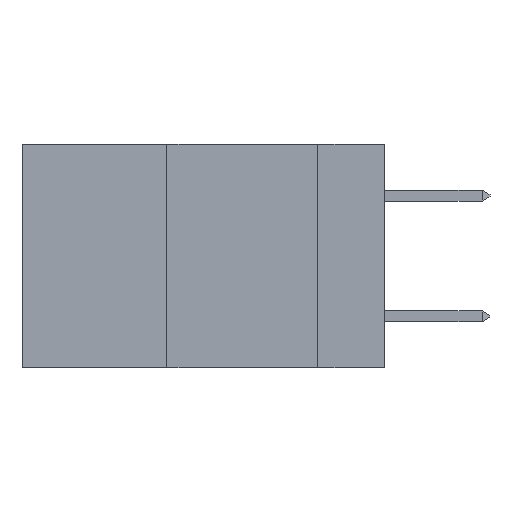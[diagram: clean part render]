
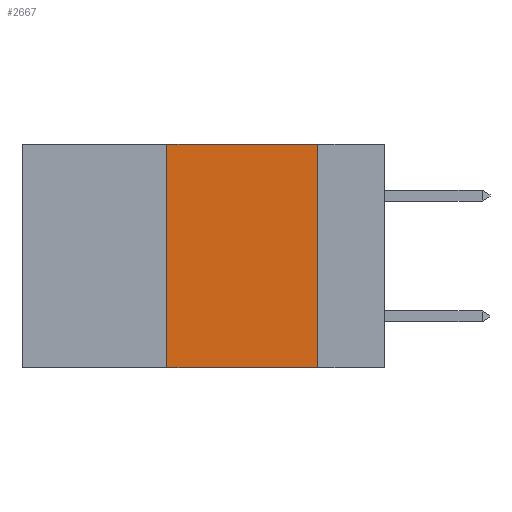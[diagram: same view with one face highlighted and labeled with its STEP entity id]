
A CAD part, left-side view. The second image highlights one B-rep face of the part: STEP entity #2667.
In plain terms, the highlighted planar face has unit normal (-1, 0, 0).
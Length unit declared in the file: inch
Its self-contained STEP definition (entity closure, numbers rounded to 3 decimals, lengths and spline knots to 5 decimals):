
#435 = LINE ( 'NONE', #2800, #4077 ) ;
#770 = AXIS2_PLACEMENT_3D ( 'NONE', #1539, #5183, #4234 ) ;
#901 = VERTEX_POINT ( 'NONE', #8192 ) ;
#927 = EDGE_CURVE ( 'NONE', #3580, #901, #435, .T. ) ;
#940 = CARTESIAN_POINT ( 'NONE',  ( 0., 0.6, 0. ) ) ;
#1525 = CARTESIAN_POINT ( 'NONE',  ( 0., 0.11, 0. ) ) ;
#1539 = CARTESIAN_POINT ( 'NONE',  ( 0., 0.6, 0. ) ) ;
#1571 = EDGE_CURVE ( 'NONE', #3580, #3682, #7435, .T. ) ;
#1695 = LINE ( 'NONE', #5953, #5404 ) ;
#1951 = ORIENTED_EDGE ( 'NONE', *, *, #7193, .F. ) ;
#2397 = PLANE ( 'NONE',  #770 ) ;
#2667 = ADVANCED_FACE ( 'NONE', ( #7418 ), #2397, .F. ) ;
#2800 = CARTESIAN_POINT ( 'NONE',  ( 0., 0.36, 0. ) ) ;
#3580 = VERTEX_POINT ( 'NONE', #7179 ) ;
#3682 = VERTEX_POINT ( 'NONE', #7223 ) ;
#3745 = VECTOR ( 'NONE', #5051, 39.37008 ) ;
#3856 = VERTEX_POINT ( 'NONE', #1525 ) ;
#3894 = ORIENTED_EDGE ( 'NONE', *, *, #1571, .T. ) ;
#4077 = VECTOR ( 'NONE', #7966, 39.37008 ) ;
#4234 = DIRECTION ( 'NONE',  ( 0., 0., -1. ) ) ;
#4501 = ORIENTED_EDGE ( 'NONE', *, *, #5436, .F. ) ;
#4643 = EDGE_LOOP ( 'NONE', ( #4501, #1951, #5954, #3894 ) ) ;
#5051 = DIRECTION ( 'NONE',  ( 0., -1., 0. ) ) ;
#5183 = DIRECTION ( 'NONE',  ( 1., 0., 0. ) ) ;
#5404 = VECTOR ( 'NONE', #7742, 39.37008 ) ;
#5436 = EDGE_CURVE ( 'NONE', #3856, #3682, #1695, .T. ) ;
#5953 = CARTESIAN_POINT ( 'NONE',  ( 0., 0.11, 0. ) ) ;
#5954 = ORIENTED_EDGE ( 'NONE', *, *, #927, .F. ) ;
#6143 = VECTOR ( 'NONE', #8703, 39.37008 ) ;
#7179 = CARTESIAN_POINT ( 'NONE',  ( 0., 0.36, -0.37 ) ) ;
#7193 = EDGE_CURVE ( 'NONE', #901, #3856, #7925, .T. ) ;
#7223 = CARTESIAN_POINT ( 'NONE',  ( 0., 0.11, -0.37 ) ) ;
#7418 = FACE_OUTER_BOUND ( 'NONE', #4643, .T. ) ;
#7435 = LINE ( 'NONE', #7762, #3745 ) ;
#7742 = DIRECTION ( 'NONE',  ( 0., 0., -1. ) ) ;
#7762 = CARTESIAN_POINT ( 'NONE',  ( 0., 0.6, -0.37 ) ) ;
#7925 = LINE ( 'NONE', #940, #6143 ) ;
#7966 = DIRECTION ( 'NONE',  ( 0., 0., 1. ) ) ;
#8192 = CARTESIAN_POINT ( 'NONE',  ( 0., 0.36, 0. ) ) ;
#8703 = DIRECTION ( 'NONE',  ( 0., -1., 0. ) ) ;
